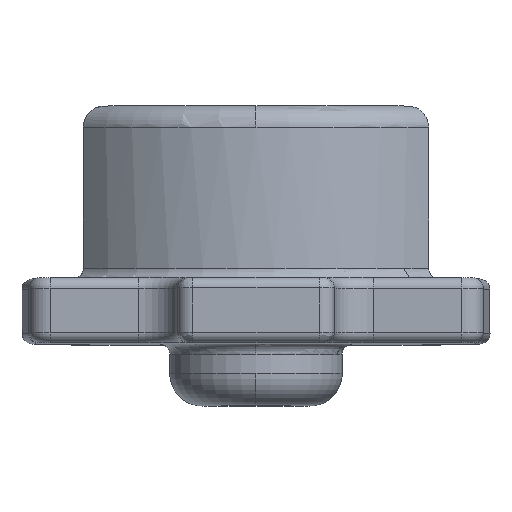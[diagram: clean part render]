
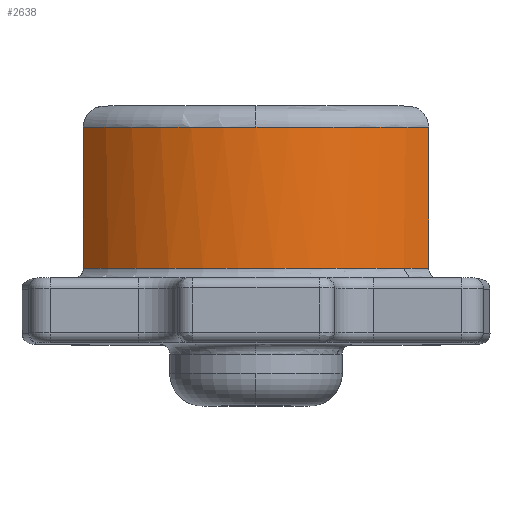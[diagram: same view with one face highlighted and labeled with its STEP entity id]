
A CAD part, top view. The second image highlights one B-rep face of the part: STEP entity #2638.
In plain terms, the highlighted cylindrical face has radius 8.255 mm (diameter 16.51 mm), a partial arc.
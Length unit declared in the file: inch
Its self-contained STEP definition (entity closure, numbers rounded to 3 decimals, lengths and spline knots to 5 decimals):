
#247=FACE_OUTER_BOUND('',#432,.T.);
#432=EDGE_LOOP('',(#2015,#2016,#2017,#2018,#2019));
#616=LINE('',#4759,#772);
#619=LINE('',#4768,#775);
#772=VECTOR('',#3554,39.37008);
#775=VECTOR('',#3565,39.37008);
#927=CIRCLE('',#2868,0.325);
#972=CIRCLE('',#2955,0.325);
#973=CIRCLE('',#2956,0.325);
#1146=VERTEX_POINT('',#4298);
#1147=VERTEX_POINT('',#4326);
#1193=VERTEX_POINT('',#4758);
#1195=VERTEX_POINT('',#4766);
#1196=VERTEX_POINT('',#4770);
#1397=EDGE_CURVE('',#1146,#1147,#927,.T.);
#1482=EDGE_CURVE('',#1193,#1146,#616,.T.);
#1487=EDGE_CURVE('',#1147,#1195,#619,.T.);
#1488=EDGE_CURVE('',#1196,#1195,#972,.T.);
#1489=EDGE_CURVE('',#1193,#1196,#973,.T.);
#2015=ORIENTED_EDGE('',*,*,#1397,.T.);
#2016=ORIENTED_EDGE('',*,*,#1487,.T.);
#2017=ORIENTED_EDGE('',*,*,#1488,.F.);
#2018=ORIENTED_EDGE('',*,*,#1489,.F.);
#2019=ORIENTED_EDGE('',*,*,#1482,.T.);
#2521=CYLINDRICAL_SURFACE('',#2954,0.325);
#2638=ADVANCED_FACE('',(#247),#2521,.T.);
#2868=AXIS2_PLACEMENT_3D('',#4343,#3366,#3367);
#2954=AXIS2_PLACEMENT_3D('',#4769,#3566,#3567);
#2955=AXIS2_PLACEMENT_3D('',#4771,#3568,#3569);
#2956=AXIS2_PLACEMENT_3D('',#4772,#3570,#3571);
#3366=DIRECTION('center_axis',(0.,1.,0.));
#3367=DIRECTION('ref_axis',(0.,0.,-1.));
#3554=DIRECTION('',(0.,-1.,0.));
#3565=DIRECTION('',(0.,1.,0.));
#3566=DIRECTION('center_axis',(0.,-1.,0.));
#3567=DIRECTION('ref_axis',(0.,0.,-1.));
#3568=DIRECTION('center_axis',(0.,1.,0.));
#3569=DIRECTION('ref_axis',(0.,0.,-1.));
#3570=DIRECTION('center_axis',(0.,1.,0.));
#3571=DIRECTION('ref_axis',(0.,0.,-1.));
#4298=CARTESIAN_POINT('',(-0.25,-8.59598,-0.91733));
#4326=CARTESIAN_POINT('',(0.25,-8.59598,-0.91733));
#4343=CARTESIAN_POINT('Origin',(0.,-8.59598,-1.125));
#4758=CARTESIAN_POINT('',(-0.25,-8.39198,-0.91733));
#4759=CARTESIAN_POINT('',(-0.25,-8.39198,-0.91733));
#4766=CARTESIAN_POINT('',(0.25,-8.39198,-0.91733));
#4768=CARTESIAN_POINT('',(0.25,-8.39198,-0.91733));
#4769=CARTESIAN_POINT('Origin',(0.,-8.39198,-1.125));
#4770=CARTESIAN_POINT('',(0.,-8.39198,-0.8));
#4771=CARTESIAN_POINT('Origin',(0.,-8.39198,-1.125));
#4772=CARTESIAN_POINT('Origin',(0.,-8.39198,-1.125));
